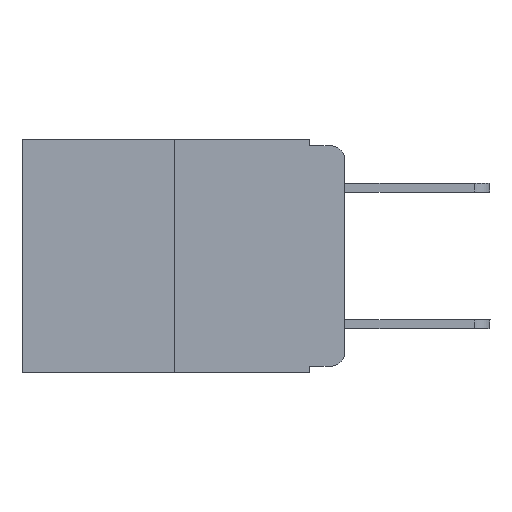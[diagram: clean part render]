
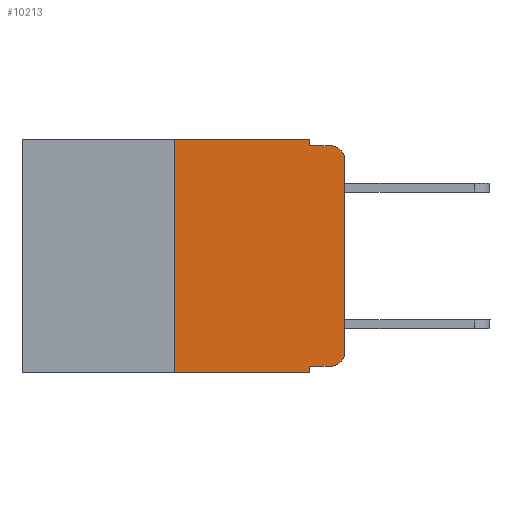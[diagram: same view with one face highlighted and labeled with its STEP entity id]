
A CAD part, left-side view. The second image highlights one B-rep face of the part: STEP entity #10213.
In plain terms, the highlighted planar face has unit normal (-1, 0, 0).
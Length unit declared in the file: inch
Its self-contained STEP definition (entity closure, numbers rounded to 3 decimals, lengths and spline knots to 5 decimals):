
#176 = VERTEX_POINT ( 'NONE', #5442 ) ;
#603 = DIRECTION ( 'NONE',  ( 0., 0., 1. ) ) ;
#665 = CARTESIAN_POINT ( 'NONE',  ( 0., 0.25, 0. ) ) ;
#952 = EDGE_CURVE ( 'NONE', #3082, #5851, #4009, .T. ) ;
#1027 = LINE ( 'NONE', #3888, #6215 ) ;
#1541 = VERTEX_POINT ( 'NONE', #665 ) ;
#1657 = DIRECTION ( 'NONE',  ( -1., 0., 0. ) ) ;
#1704 = LINE ( 'NONE', #9399, #2384 ) ;
#1812 = DIRECTION ( 'NONE',  ( 0., -1., 0. ) ) ;
#2179 = ORIENTED_EDGE ( 'NONE', *, *, #9601, .T. ) ;
#2273 = VERTEX_POINT ( 'NONE', #5083 ) ;
#2384 = VECTOR ( 'NONE', #8663, 39.37008 ) ;
#2411 = DIRECTION ( 'NONE',  ( 0., 0., -1. ) ) ;
#2511 = DIRECTION ( 'NONE',  ( 0., 0., -1. ) ) ;
#2611 = VERTEX_POINT ( 'NONE', #6597 ) ;
#2656 = DIRECTION ( 'NONE',  ( 1., 0., 0. ) ) ;
#2845 = CIRCLE ( 'NONE', #6046, 0.02 ) ;
#3082 = VERTEX_POINT ( 'NONE', #8505 ) ;
#3349 = LINE ( 'NONE', #9613, #9527 ) ;
#3437 = ORIENTED_EDGE ( 'NONE', *, *, #4269, .T. ) ;
#3763 = EDGE_CURVE ( 'NONE', #7507, #8231, #3349, .T. ) ;
#3854 = CARTESIAN_POINT ( 'NONE',  ( 0., 0.051, -0.333 ) ) ;
#3888 = CARTESIAN_POINT ( 'NONE',  ( 0., 0.473, -0.343 ) ) ;
#4000 = CARTESIAN_POINT ( 'NONE',  ( 0., 0.02, -0.333 ) ) ;
#4009 = LINE ( 'NONE', #4054, #11012 ) ;
#4054 = CARTESIAN_POINT ( 'NONE',  ( 0., 0., 0. ) ) ;
#4059 = CARTESIAN_POINT ( 'NONE',  ( 0., 0., -0.03 ) ) ;
#4269 = EDGE_CURVE ( 'NONE', #2273, #6313, #1027, .T. ) ;
#4548 = LINE ( 'NONE', #9190, #6903 ) ;
#4979 = ORIENTED_EDGE ( 'NONE', *, *, #10761, .T. ) ;
#5083 = CARTESIAN_POINT ( 'NONE',  ( 0., 0.25, -0.343 ) ) ;
#5153 = DIRECTION ( 'NONE',  ( 0., -1., 0. ) ) ;
#5352 = CARTESIAN_POINT ( 'NONE',  ( 0., 0.473, 0. ) ) ;
#5442 = CARTESIAN_POINT ( 'NONE',  ( 0., 0.02, -0.01 ) ) ;
#5492 = CARTESIAN_POINT ( 'NONE',  ( 0., 0.02, -0.03 ) ) ;
#5574 = LINE ( 'NONE', #3854, #11204 ) ;
#5593 = DIRECTION ( 'NONE',  ( 0., 0., 1. ) ) ;
#5851 = VERTEX_POINT ( 'NONE', #4059 ) ;
#6007 = ORIENTED_EDGE ( 'NONE', *, *, #952, .T. ) ;
#6037 = ORIENTED_EDGE ( 'NONE', *, *, #6340, .T. ) ;
#6046 = AXIS2_PLACEMENT_3D ( 'NONE', #5492, #9166, #10736 ) ;
#6215 = VECTOR ( 'NONE', #5153, 39.37008 ) ;
#6313 = VERTEX_POINT ( 'NONE', #10082 ) ;
#6340 = EDGE_CURVE ( 'NONE', #2611, #8515, #5574, .T. ) ;
#6561 = EDGE_LOOP ( 'NONE', ( #6007, #2179, #10794, #11155, #10351, #8942, #3437, #7486, #6037, #4979 ) ) ;
#6597 = CARTESIAN_POINT ( 'NONE',  ( 0., 0.051, -0.333 ) ) ;
#6668 = DIRECTION ( 'NONE',  ( 0., -1., 0. ) ) ;
#6864 = CARTESIAN_POINT ( 'NONE',  ( 0., 0.051, 0. ) ) ;
#6903 = VECTOR ( 'NONE', #5593, 39.37008 ) ;
#6934 = LINE ( 'NONE', #11179, #8562 ) ;
#6976 = CIRCLE ( 'NONE', #10884, 0.02 ) ;
#7486 = ORIENTED_EDGE ( 'NONE', *, *, #7581, .F. ) ;
#7507 = VERTEX_POINT ( 'NONE', #6864 ) ;
#7581 = EDGE_CURVE ( 'NONE', #2611, #6313, #6934, .T. ) ;
#7821 = DIRECTION ( 'NONE',  ( 0., 0., -1. ) ) ;
#7939 = LINE ( 'NONE', #5352, #10413 ) ;
#7954 = EDGE_CURVE ( 'NONE', #8231, #176, #1704, .T. ) ;
#8231 = VERTEX_POINT ( 'NONE', #8894 ) ;
#8330 = EDGE_CURVE ( 'NONE', #2273, #1541, #4548, .T. ) ;
#8505 = CARTESIAN_POINT ( 'NONE',  ( 0., 0., -0.313 ) ) ;
#8515 = VERTEX_POINT ( 'NONE', #4000 ) ;
#8562 = VECTOR ( 'NONE', #2411, 39.37008 ) ;
#8663 = DIRECTION ( 'NONE',  ( 0., -1., 0. ) ) ;
#8795 = PLANE ( 'NONE',  #11038 ) ;
#8827 = DIRECTION ( 'NONE',  ( 0., 0., -1. ) ) ;
#8894 = CARTESIAN_POINT ( 'NONE',  ( 0., 0.051, -0.01 ) ) ;
#8942 = ORIENTED_EDGE ( 'NONE', *, *, #8330, .F. ) ;
#9166 = DIRECTION ( 'NONE',  ( -1., 0., 0. ) ) ;
#9190 = CARTESIAN_POINT ( 'NONE',  ( 0., 0.25, 0. ) ) ;
#9399 = CARTESIAN_POINT ( 'NONE',  ( 0., 0.051, -0.01 ) ) ;
#9527 = VECTOR ( 'NONE', #2511, 39.37008 ) ;
#9601 = EDGE_CURVE ( 'NONE', #5851, #176, #2845, .T. ) ;
#9613 = CARTESIAN_POINT ( 'NONE',  ( 0., 0.051, 0. ) ) ;
#9677 = CARTESIAN_POINT ( 'NONE',  ( 0., 0.02, -0.313 ) ) ;
#10082 = CARTESIAN_POINT ( 'NONE',  ( 0., 0.051, -0.343 ) ) ;
#10127 = FACE_OUTER_BOUND ( 'NONE', #6561, .T. ) ;
#10213 = ADVANCED_FACE ( 'NONE', ( #10127 ), #8795, .F. ) ;
#10234 = EDGE_CURVE ( 'NONE', #1541, #7507, #7939, .T. ) ;
#10351 = ORIENTED_EDGE ( 'NONE', *, *, #10234, .F. ) ;
#10413 = VECTOR ( 'NONE', #1812, 39.37008 ) ;
#10670 = CARTESIAN_POINT ( 'NONE',  ( 0., 0.473, 0. ) ) ;
#10736 = DIRECTION ( 'NONE',  ( 0., 0., -1. ) ) ;
#10761 = EDGE_CURVE ( 'NONE', #8515, #3082, #6976, .T. ) ;
#10794 = ORIENTED_EDGE ( 'NONE', *, *, #7954, .F. ) ;
#10884 = AXIS2_PLACEMENT_3D ( 'NONE', #9677, #1657, #7821 ) ;
#11012 = VECTOR ( 'NONE', #603, 39.37008 ) ;
#11038 = AXIS2_PLACEMENT_3D ( 'NONE', #10670, #2656, #8827 ) ;
#11155 = ORIENTED_EDGE ( 'NONE', *, *, #3763, .F. ) ;
#11179 = CARTESIAN_POINT ( 'NONE',  ( 0., 0.051, 0. ) ) ;
#11204 = VECTOR ( 'NONE', #6668, 39.37008 ) ;
